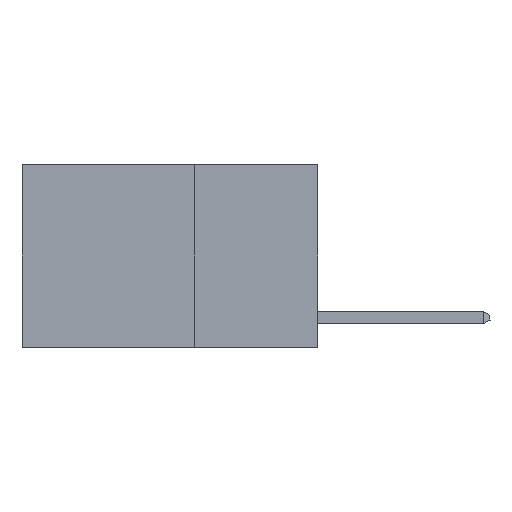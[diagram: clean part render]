
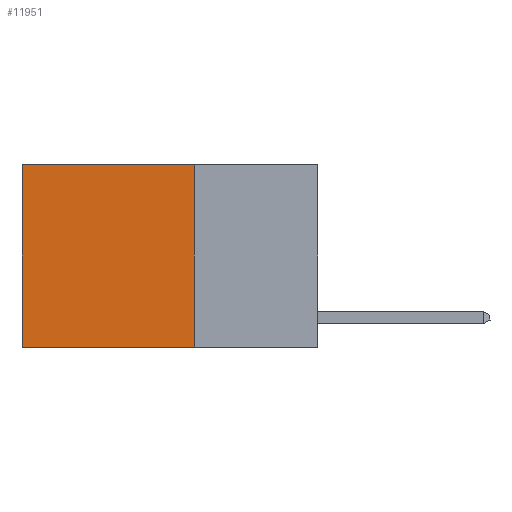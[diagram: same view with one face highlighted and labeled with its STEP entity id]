
A CAD part, left-side view. The second image highlights one B-rep face of the part: STEP entity #11951.
In plain terms, the highlighted planar face has unit normal (-1, 0, 0).
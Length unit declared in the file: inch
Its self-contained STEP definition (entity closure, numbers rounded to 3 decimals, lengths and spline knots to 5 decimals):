
#1892 = VERTEX_POINT ( 'NONE', #3997 ) ;
#2018 = VECTOR ( 'NONE', #8685, 39.37008 ) ;
#2440 = CARTESIAN_POINT ( 'NONE',  ( 0.2625, 0.6, 0. ) ) ;
#2619 = CARTESIAN_POINT ( 'NONE',  ( 0.2625, 0.25, 0. ) ) ;
#2697 = VECTOR ( 'NONE', #11214, 39.37008 ) ;
#2951 = CARTESIAN_POINT ( 'NONE',  ( 0.2625, 0.25, 0. ) ) ;
#2975 = VERTEX_POINT ( 'NONE', #13932 ) ;
#3115 = ORIENTED_EDGE ( 'NONE', *, *, #9042, .F. ) ;
#3624 = CARTESIAN_POINT ( 'NONE',  ( 0.2625, 0.6, -0.37 ) ) ;
#3997 = CARTESIAN_POINT ( 'NONE',  ( 0.2625, 0.25, 0. ) ) ;
#4217 = VERTEX_POINT ( 'NONE', #3624 ) ;
#4382 = DIRECTION ( 'NONE',  ( 0., 0., -1. ) ) ;
#5883 = LINE ( 'NONE', #18753, #2018 ) ;
#6056 = ORIENTED_EDGE ( 'NONE', *, *, #9958, .T. ) ;
#6227 = LINE ( 'NONE', #2619, #9225 ) ;
#6513 = ORIENTED_EDGE ( 'NONE', *, *, #18126, .F. ) ;
#7253 = LINE ( 'NONE', #7961, #18782 ) ;
#7961 = CARTESIAN_POINT ( 'NONE',  ( 0.2625, 0.25, 0. ) ) ;
#8141 = AXIS2_PLACEMENT_3D ( 'NONE', #2951, #13091, #4382 ) ;
#8685 = DIRECTION ( 'NONE',  ( 0., 1., 0. ) ) ;
#9042 = EDGE_CURVE ( 'NONE', #1892, #2975, #6227, .T. ) ;
#9225 = VECTOR ( 'NONE', #11325, 39.37008 ) ;
#9950 = VERTEX_POINT ( 'NONE', #2440 ) ;
#9958 = EDGE_CURVE ( 'NONE', #9950, #4217, #17652, .T. ) ;
#11214 = DIRECTION ( 'NONE',  ( 0., 0., -1. ) ) ;
#11325 = DIRECTION ( 'NONE',  ( 0., 0., -1. ) ) ;
#11687 = FACE_OUTER_BOUND ( 'NONE', #15767, .T. ) ;
#11951 = ADVANCED_FACE ( 'NONE', ( #11687 ), #15946, .F. ) ;
#13091 = DIRECTION ( 'NONE',  ( 1., 0., 0. ) ) ;
#13932 = CARTESIAN_POINT ( 'NONE',  ( 0.2625, 0.25, -0.37 ) ) ;
#15767 = EDGE_LOOP ( 'NONE', ( #6056, #6513, #3115, #18503 ) ) ;
#15946 = PLANE ( 'NONE',  #8141 ) ;
#16633 = DIRECTION ( 'NONE',  ( 0., 1., 0. ) ) ;
#16952 = CARTESIAN_POINT ( 'NONE',  ( 0.2625, 0.6, 0. ) ) ;
#17652 = LINE ( 'NONE', #16952, #2697 ) ;
#18126 = EDGE_CURVE ( 'NONE', #2975, #4217, #5883, .T. ) ;
#18503 = ORIENTED_EDGE ( 'NONE', *, *, #18701, .T. ) ;
#18701 = EDGE_CURVE ( 'NONE', #1892, #9950, #7253, .T. ) ;
#18753 = CARTESIAN_POINT ( 'NONE',  ( 0.2625, 0.25, -0.37 ) ) ;
#18782 = VECTOR ( 'NONE', #16633, 39.37008 ) ;
